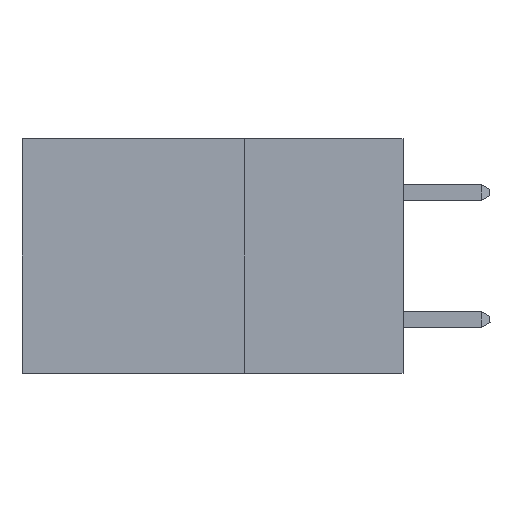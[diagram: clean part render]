
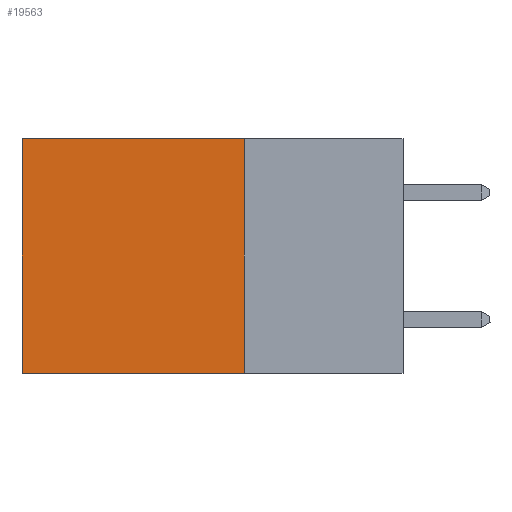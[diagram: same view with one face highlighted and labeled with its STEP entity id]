
A CAD part, left-side view. The second image highlights one B-rep face of the part: STEP entity #19563.
In plain terms, the highlighted planar face has unit normal (-1, 0, 0).
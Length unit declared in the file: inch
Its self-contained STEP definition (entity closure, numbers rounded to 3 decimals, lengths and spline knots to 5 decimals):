
#113 = EDGE_CURVE ( 'NONE', #33085, #20832, #30947, .T. ) ;
#571 = VERTEX_POINT ( 'NONE', #8947 ) ;
#2391 = DIRECTION ( 'NONE',  ( 0., 0., -1. ) ) ;
#3864 = AXIS2_PLACEMENT_3D ( 'NONE', #22584, #38527, #18841 ) ;
#4220 = DIRECTION ( 'NONE',  ( 0., 0., -1. ) ) ;
#4381 = EDGE_CURVE ( 'NONE', #30977, #571, #26003, .T. ) ;
#5272 = VECTOR ( 'NONE', #13520, 39.37008 ) ;
#5479 = ORIENTED_EDGE ( 'NONE', *, *, #113, .F. ) ;
#6358 = ORIENTED_EDGE ( 'NONE', *, *, #4381, .T. ) ;
#8947 = CARTESIAN_POINT ( 'NONE',  ( 0.2875, 0.6, -0.37 ) ) ;
#11057 = CARTESIAN_POINT ( 'NONE',  ( 0.2875, 0.6, 0. ) ) ;
#13468 = EDGE_LOOP ( 'NONE', ( #6358, #16711, #5479, #21094 ) ) ;
#13520 = DIRECTION ( 'NONE',  ( 0., 1., 0. ) ) ;
#16521 = CARTESIAN_POINT ( 'NONE',  ( 0.2875, 0.25, -0.37 ) ) ;
#16711 = ORIENTED_EDGE ( 'NONE', *, *, #40169, .F. ) ;
#16790 = FACE_OUTER_BOUND ( 'NONE', #13468, .T. ) ;
#17241 = VECTOR ( 'NONE', #4220, 39.37008 ) ;
#17679 = LINE ( 'NONE', #16521, #5272 ) ;
#17724 = LINE ( 'NONE', #24216, #24904 ) ;
#18841 = DIRECTION ( 'NONE',  ( 0., 0., -1. ) ) ;
#19563 = ADVANCED_FACE ( 'NONE', ( #16790 ), #22005, .F. ) ;
#20832 = VERTEX_POINT ( 'NONE', #25481 ) ;
#21094 = ORIENTED_EDGE ( 'NONE', *, *, #30024, .T. ) ;
#22005 = PLANE ( 'NONE',  #3864 ) ;
#22584 = CARTESIAN_POINT ( 'NONE',  ( 0.2875, 0.25, 0. ) ) ;
#23632 = DIRECTION ( 'NONE',  ( 0., 1., 0. ) ) ;
#24216 = CARTESIAN_POINT ( 'NONE',  ( 0.2875, 0.25, 0. ) ) ;
#24904 = VECTOR ( 'NONE', #23632, 39.37008 ) ;
#25481 = CARTESIAN_POINT ( 'NONE',  ( 0.2875, 0.25, -0.37 ) ) ;
#26003 = LINE ( 'NONE', #27577, #17241 ) ;
#27353 = VECTOR ( 'NONE', #2391, 39.37008 ) ;
#27577 = CARTESIAN_POINT ( 'NONE',  ( 0.2875, 0.6, 0. ) ) ;
#28776 = CARTESIAN_POINT ( 'NONE',  ( 0.2875, 0.25, 0. ) ) ;
#30024 = EDGE_CURVE ( 'NONE', #33085, #30977, #17724, .T. ) ;
#30947 = LINE ( 'NONE', #28776, #27353 ) ;
#30977 = VERTEX_POINT ( 'NONE', #11057 ) ;
#32122 = CARTESIAN_POINT ( 'NONE',  ( 0.2875, 0.25, 0. ) ) ;
#33085 = VERTEX_POINT ( 'NONE', #32122 ) ;
#38527 = DIRECTION ( 'NONE',  ( 1., 0., 0. ) ) ;
#40169 = EDGE_CURVE ( 'NONE', #20832, #571, #17679, .T. ) ;
